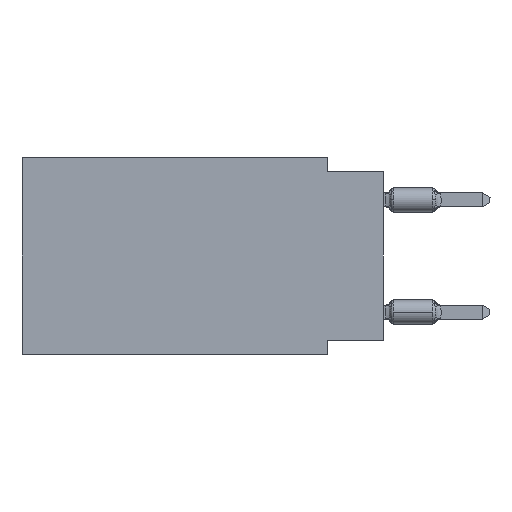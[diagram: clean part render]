
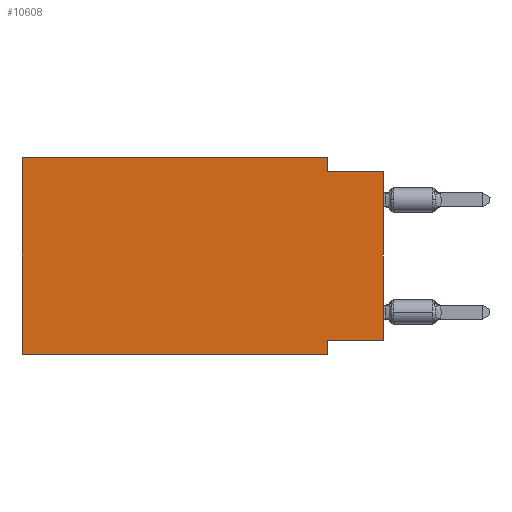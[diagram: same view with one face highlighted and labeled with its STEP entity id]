
A CAD part, left-side view. The second image highlights one B-rep face of the part: STEP entity #10608.
In plain terms, the highlighted planar face has unit normal (-1, 0, 0).
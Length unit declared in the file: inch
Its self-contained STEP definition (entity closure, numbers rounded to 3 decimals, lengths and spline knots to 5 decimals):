
#407 = DIRECTION ( 'NONE',  ( 0., 0., -1. ) ) ;
#556 = EDGE_CURVE ( 'NONE', #14756, #26256, #15597, .T. ) ;
#677 = ORIENTED_EDGE ( 'NONE', *, *, #15935, .F. ) ;
#1446 = CARTESIAN_POINT ( 'NONE',  ( 0., 0.1, -0.325 ) ) ;
#1641 = LINE ( 'NONE', #8590, #4052 ) ;
#1939 = VECTOR ( 'NONE', #14270, 39.37008 ) ;
#2064 = DIRECTION ( 'NONE',  ( 0., 0., -1. ) ) ;
#2089 = CARTESIAN_POINT ( 'NONE',  ( 0., 0.645, -0.35 ) ) ;
#2248 = EDGE_CURVE ( 'NONE', #14522, #26460, #24290, .T. ) ;
#2779 = PLANE ( 'NONE',  #26174 ) ;
#3803 = VERTEX_POINT ( 'NONE', #5969 ) ;
#4003 = ORIENTED_EDGE ( 'NONE', *, *, #23683, .F. ) ;
#4052 = VECTOR ( 'NONE', #6073, 39.37008 ) ;
#4260 = CARTESIAN_POINT ( 'NONE',  ( 0., 0.1, 0. ) ) ;
#4995 = FACE_OUTER_BOUND ( 'NONE', #12739, .T. ) ;
#5963 = VERTEX_POINT ( 'NONE', #1446 ) ;
#5966 = DIRECTION ( 'NONE',  ( 0., 0., 1. ) ) ;
#5969 = CARTESIAN_POINT ( 'NONE',  ( 0., 0.1, -0.025 ) ) ;
#6073 = DIRECTION ( 'NONE',  ( 0., -1., 0. ) ) ;
#6705 = EDGE_CURVE ( 'NONE', #3803, #26256, #1641, .T. ) ;
#8590 = CARTESIAN_POINT ( 'NONE',  ( 0., 0., -0.025 ) ) ;
#8910 = CARTESIAN_POINT ( 'NONE',  ( 0., 0., -0.325 ) ) ;
#8975 = CARTESIAN_POINT ( 'NONE',  ( 0., 0., -0.025 ) ) ;
#9370 = VECTOR ( 'NONE', #9947, 39.37008 ) ;
#9947 = DIRECTION ( 'NONE',  ( 0., 1., 0. ) ) ;
#10163 = CARTESIAN_POINT ( 'NONE',  ( 0., 0., -0.325 ) ) ;
#10608 = ADVANCED_FACE ( 'NONE', ( #4995 ), #2779, .F. ) ;
#11651 = ORIENTED_EDGE ( 'NONE', *, *, #28644, .F. ) ;
#11978 = EDGE_CURVE ( 'NONE', #14522, #22335, #26193, .T. ) ;
#12235 = CARTESIAN_POINT ( 'NONE',  ( 0., 0.645, 0. ) ) ;
#12321 = LINE ( 'NONE', #8910, #9370 ) ;
#12440 = CARTESIAN_POINT ( 'NONE',  ( 0., 0.645, 0. ) ) ;
#12739 = EDGE_LOOP ( 'NONE', ( #21330, #13582, #4003, #15017, #20211, #22801, #677, #11651 ) ) ;
#13054 = VECTOR ( 'NONE', #14450, 39.37008 ) ;
#13553 = CARTESIAN_POINT ( 'NONE',  ( 0., 0., 0. ) ) ;
#13582 = ORIENTED_EDGE ( 'NONE', *, *, #6705, .F. ) ;
#14270 = DIRECTION ( 'NONE',  ( 0., -1., 0. ) ) ;
#14450 = DIRECTION ( 'NONE',  ( 0., 0., 1. ) ) ;
#14522 = VERTEX_POINT ( 'NONE', #29872 ) ;
#14756 = VERTEX_POINT ( 'NONE', #10163 ) ;
#15017 = ORIENTED_EDGE ( 'NONE', *, *, #16629, .F. ) ;
#15597 = LINE ( 'NONE', #13553, #30349 ) ;
#15935 = EDGE_CURVE ( 'NONE', #5963, #22335, #17260, .T. ) ;
#16629 = EDGE_CURVE ( 'NONE', #26460, #17546, #23960, .T. ) ;
#17260 = LINE ( 'NONE', #26936, #22792 ) ;
#17546 = VERTEX_POINT ( 'NONE', #20411 ) ;
#18268 = VECTOR ( 'NONE', #24060, 39.37008 ) ;
#20211 = ORIENTED_EDGE ( 'NONE', *, *, #2248, .F. ) ;
#20411 = CARTESIAN_POINT ( 'NONE',  ( 0., 0.1, 0. ) ) ;
#20868 = DIRECTION ( 'NONE',  ( 0., -1., 0. ) ) ;
#21330 = ORIENTED_EDGE ( 'NONE', *, *, #556, .T. ) ;
#21379 = LINE ( 'NONE', #4260, #18268 ) ;
#22128 = DIRECTION ( 'NONE',  ( 1., 0., 0. ) ) ;
#22335 = VERTEX_POINT ( 'NONE', #24713 ) ;
#22792 = VECTOR ( 'NONE', #2064, 39.37008 ) ;
#22801 = ORIENTED_EDGE ( 'NONE', *, *, #11978, .T. ) ;
#23683 = EDGE_CURVE ( 'NONE', #17546, #3803, #21379, .T. ) ;
#23960 = LINE ( 'NONE', #28173, #25835 ) ;
#24060 = DIRECTION ( 'NONE',  ( 0., 0., -1. ) ) ;
#24189 = CARTESIAN_POINT ( 'NONE',  ( 0., 0.645, 0. ) ) ;
#24290 = LINE ( 'NONE', #12235, #13054 ) ;
#24713 = CARTESIAN_POINT ( 'NONE',  ( 0., 0.1, -0.35 ) ) ;
#25835 = VECTOR ( 'NONE', #20868, 39.37008 ) ;
#26174 = AXIS2_PLACEMENT_3D ( 'NONE', #12440, #22128, #407 ) ;
#26193 = LINE ( 'NONE', #2089, #1939 ) ;
#26256 = VERTEX_POINT ( 'NONE', #8975 ) ;
#26460 = VERTEX_POINT ( 'NONE', #24189 ) ;
#26936 = CARTESIAN_POINT ( 'NONE',  ( 0., 0.1, -0.35 ) ) ;
#28173 = CARTESIAN_POINT ( 'NONE',  ( 0., 0.645, 0. ) ) ;
#28644 = EDGE_CURVE ( 'NONE', #14756, #5963, #12321, .T. ) ;
#29872 = CARTESIAN_POINT ( 'NONE',  ( 0., 0.645, -0.35 ) ) ;
#30349 = VECTOR ( 'NONE', #5966, 39.37008 ) ;
